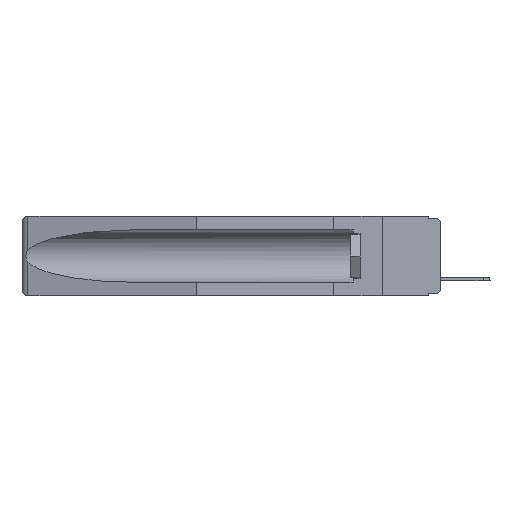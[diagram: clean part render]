
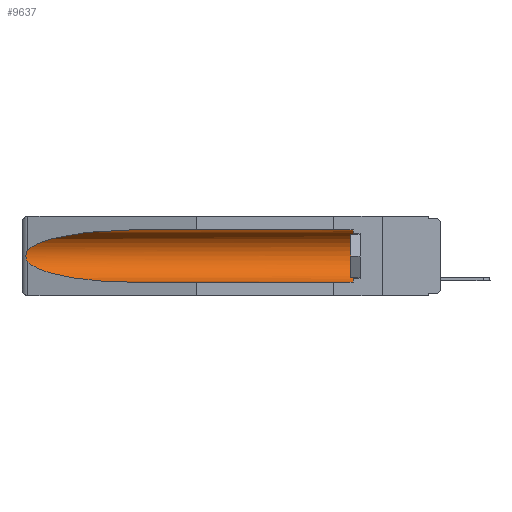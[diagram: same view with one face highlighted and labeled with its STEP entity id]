
A CAD part, left-side view. The second image highlights one B-rep face of the part: STEP entity #9637.
In plain terms, the highlighted cylindrical face has radius 2.857 mm (diameter 5.715 mm), a partial arc.
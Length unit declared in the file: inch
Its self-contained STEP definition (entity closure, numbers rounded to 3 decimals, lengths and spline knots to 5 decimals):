
#756 = CARTESIAN_POINT ( 'NONE',  ( 0.26537, 1.52718, -0.14972 ) ) ;
#1061 = DIRECTION ( 'NONE',  ( 0., 1., 0. ) ) ;
#1734 = EDGE_CURVE ( 'NONE', #19711, #8641, #10545, .T. ) ;
#1802 = EDGE_CURVE ( 'NONE', #15411, #8641, #4906, .T. ) ;
#2024 = CARTESIAN_POINT ( 'NONE',  ( 0.155, 1.07973, -0.059 ) ) ;
#2155 = EDGE_CURVE ( 'NONE', #11483, #15411, #16441, .T. ) ;
#2352 = EDGE_CURVE ( 'NONE', #19711, #12491, #7888, .T. ) ;
#2964 = CARTESIAN_POINT ( 'NONE',  ( 0.26537, 1.52718, -0.19328 ) ) ;
#3805 = CARTESIAN_POINT ( 'NONE',  ( 0.2673, 1.53269, -0.17917 ) ) ;
#3826 = CARTESIAN_POINT ( 'NONE',  ( 0.155, -0.30754, -0.284 ) ) ;
#4646 = CARTESIAN_POINT ( 'NONE',  ( 0.155, 1.07973, -0.284 ) ) ;
#4906 =( BOUNDED_CURVE ( )  B_SPLINE_CURVE ( 3, ( #2964, #18826, #17233, #4646 ),
 .UNSPECIFIED., .F., .T. ) 
 B_SPLINE_CURVE_WITH_KNOTS ( ( 4, 4 ),
 ( 0.1948, 1.5708 ),
 .UNSPECIFIED. ) 
 CURVE ( )  GEOMETRIC_REPRESENTATION_ITEM ( )  RATIONAL_B_SPLINE_CURVE ( ( 1., 0.848, 0.848, 1. ) ) 
 REPRESENTATION_ITEM ( '' )  );
#5428 = CARTESIAN_POINT ( 'NONE',  ( 0.21114, 1.30732, -0.059 ) ) ;
#5520 = CARTESIAN_POINT ( 'NONE',  ( 0.155, 1.07973, -0.059 ) ) ;
#5603 = CARTESIAN_POINT ( 'NONE',  ( 0.155, -0.30754, -0.059 ) ) ;
#6014 = VECTOR ( 'NONE', #15114, 39.37008 ) ;
#6314 = ORIENTED_EDGE ( 'NONE', *, *, #2155, .T. ) ;
#6789 = ORIENTED_EDGE ( 'NONE', *, *, #16396, .T. ) ;
#6961 = CARTESIAN_POINT ( 'NONE',  ( 0.26654, 1.53092, -0.15636 ) ) ;
#7640 = ORIENTED_EDGE ( 'NONE', *, *, #2352, .T. ) ;
#7846 = VECTOR ( 'NONE', #1061, 39.37008 ) ;
#7888 = CIRCLE ( 'NONE', #13294, 0.1125 ) ;
#8439 = CARTESIAN_POINT ( 'NONE',  ( 0.155, 0.126, -0.1715 ) ) ;
#8641 = VERTEX_POINT ( 'NONE', #12861 ) ;
#8659 = CARTESIAN_POINT ( 'NONE',  ( 0.26537, 1.52718, -0.19328 ) ) ;
#9464 = CARTESIAN_POINT ( 'NONE',  ( 0.155, 0.126, -0.284 ) ) ;
#9637 = ADVANCED_FACE ( 'NONE', ( #9744 ), #19803, .F. ) ;
#9744 = FACE_OUTER_BOUND ( 'NONE', #16383, .T. ) ;
#9796 = ORIENTED_EDGE ( 'NONE', *, *, #1734, .F. ) ;
#10067 = CARTESIAN_POINT ( 'NONE',  ( 0.155, -0.30754, -0.1715 ) ) ;
#10227 = CARTESIAN_POINT ( 'NONE',  ( 0.26655, 1.53094, -0.18657 ) ) ;
#10545 = LINE ( 'NONE', #3826, #7846 ) ;
#11483 = VERTEX_POINT ( 'NONE', #17317 ) ;
#12151 = LINE ( 'NONE', #5603, #6014 ) ;
#12163 = EDGE_CURVE ( 'NONE', #20816, #11483, #20164, .T. ) ;
#12491 = VERTEX_POINT ( 'NONE', #17895 ) ;
#12861 = CARTESIAN_POINT ( 'NONE',  ( 0.155, 1.07973, -0.284 ) ) ;
#13182 = DIRECTION ( 'NONE',  ( 0., 0., 1. ) ) ;
#13294 = AXIS2_PLACEMENT_3D ( 'NONE', #8439, #20907, #13182 ) ;
#13405 = CARTESIAN_POINT ( 'NONE',  ( 0.2673, 1.5327, -0.16383 ) ) ;
#13431 = AXIS2_PLACEMENT_3D ( 'NONE', #10067, #18233, #16725 ) ;
#15030 = CARTESIAN_POINT ( 'NONE',  ( 0.25451, 1.48313, -0.09465 ) ) ;
#15114 = DIRECTION ( 'NONE',  ( 0., 1., 0. ) ) ;
#15301 = CARTESIAN_POINT ( 'NONE',  ( 0.2675, 1.53308, -0.17534 ) ) ;
#15411 = VERTEX_POINT ( 'NONE', #19524 ) ;
#16383 = EDGE_LOOP ( 'NONE', ( #20829, #6314, #17855, #9796, #7640, #6789 ) ) ;
#16396 = EDGE_CURVE ( 'NONE', #12491, #20816, #12151, .T. ) ;
#16441 = B_SPLINE_CURVE_WITH_KNOTS ( 'NONE', 3,
 ( #16899, #16993, #6961, #13405, #18295, #15301, #3805, #10227, #16691, #8659 ),
 .UNSPECIFIED., .F., .F.,
 ( 4, 2, 2, 2, 4 ),
 ( 0., 0.00029, 0.00058, 0.00087, 0.00117 ),
 .UNSPECIFIED. ) ;
#16691 = CARTESIAN_POINT ( 'NONE',  ( 0.26597, 1.5296, -0.19026 ) ) ;
#16725 = DIRECTION ( 'NONE',  ( 0., 0., 1. ) ) ;
#16899 = CARTESIAN_POINT ( 'NONE',  ( 0.26537, 1.52718, -0.14972 ) ) ;
#16993 = CARTESIAN_POINT ( 'NONE',  ( 0.26597, 1.52961, -0.15275 ) ) ;
#17233 = CARTESIAN_POINT ( 'NONE',  ( 0.21114, 1.30732, -0.284 ) ) ;
#17317 = CARTESIAN_POINT ( 'NONE',  ( 0.26537, 1.52718, -0.14972 ) ) ;
#17855 = ORIENTED_EDGE ( 'NONE', *, *, #1802, .T. ) ;
#17895 = CARTESIAN_POINT ( 'NONE',  ( 0.155, 0.126, -0.059 ) ) ;
#18233 = DIRECTION ( 'NONE',  ( 0., 1., 0. ) ) ;
#18295 = CARTESIAN_POINT ( 'NONE',  ( 0.2675, 1.53308, -0.16763 ) ) ;
#18826 = CARTESIAN_POINT ( 'NONE',  ( 0.25451, 1.48313, -0.24835 ) ) ;
#19524 = CARTESIAN_POINT ( 'NONE',  ( 0.26537, 1.52718, -0.19328 ) ) ;
#19711 = VERTEX_POINT ( 'NONE', #9464 ) ;
#19803 = CYLINDRICAL_SURFACE ( 'NONE', #13431, 0.1125 ) ;
#20164 =( BOUNDED_CURVE ( )  B_SPLINE_CURVE ( 3, ( #5520, #5428, #15030, #756 ),
 .UNSPECIFIED., .F., .F. ) 
 B_SPLINE_CURVE_WITH_KNOTS ( ( 4, 4 ),
 ( 4.71239, 6.08839 ),
 .UNSPECIFIED. ) 
 CURVE ( )  GEOMETRIC_REPRESENTATION_ITEM ( )  RATIONAL_B_SPLINE_CURVE ( ( 1., 0.848, 0.848, 1. ) ) 
 REPRESENTATION_ITEM ( '' )  );
#20816 = VERTEX_POINT ( 'NONE', #2024 ) ;
#20829 = ORIENTED_EDGE ( 'NONE', *, *, #12163, .T. ) ;
#20907 = DIRECTION ( 'NONE',  ( 0., -1., 0. ) ) ;
